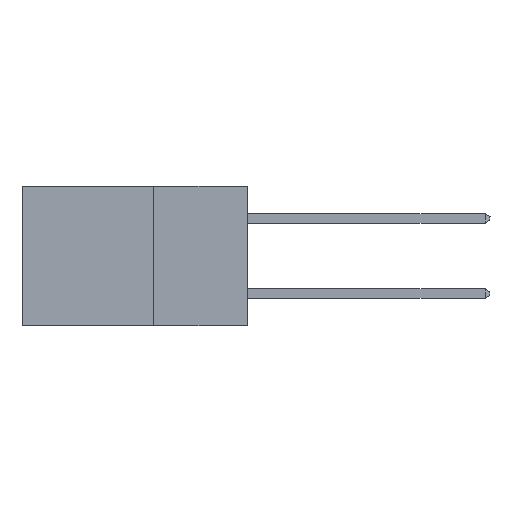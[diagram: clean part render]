
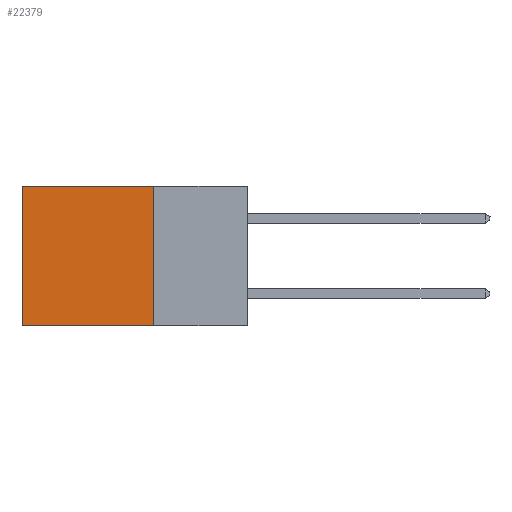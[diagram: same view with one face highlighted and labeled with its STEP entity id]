
A CAD part, left-side view. The second image highlights one B-rep face of the part: STEP entity #22379.
In plain terms, the highlighted planar face has unit normal (-1, 0, 0).
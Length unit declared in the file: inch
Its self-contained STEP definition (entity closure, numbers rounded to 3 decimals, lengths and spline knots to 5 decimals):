
#1244 = VERTEX_POINT ( 'NONE', #3478 ) ;
#1535 = DIRECTION ( 'NONE',  ( 0., 1., 0. ) ) ;
#2784 = AXIS2_PLACEMENT_3D ( 'NONE', #3380, #22066, #13731 ) ;
#3104 = EDGE_CURVE ( 'NONE', #1244, #11530, #9121, .T. ) ;
#3380 = CARTESIAN_POINT ( 'NONE',  ( 0.2615, 0.25, -0.37 ) ) ;
#3478 = CARTESIAN_POINT ( 'NONE',  ( 0.2615, 0.25, 0. ) ) ;
#4189 = DIRECTION ( 'NONE',  ( 0., 1., 0. ) ) ;
#4987 = LINE ( 'NONE', #11821, #6689 ) ;
#5303 = EDGE_LOOP ( 'NONE', ( #19051, #20896, #7259, #17029 ) ) ;
#5463 = DIRECTION ( 'NONE',  ( 0., 0., -1. ) ) ;
#6643 = LINE ( 'NONE', #10264, #13486 ) ;
#6689 = VECTOR ( 'NONE', #22068, 39.37008 ) ;
#7259 = ORIENTED_EDGE ( 'NONE', *, *, #3104, .F. ) ;
#7707 = LINE ( 'NONE', #18281, #16753 ) ;
#8409 = PLANE ( 'NONE',  #2784 ) ;
#8454 = CARTESIAN_POINT ( 'NONE',  ( 0.2615, 0.25, -0.37 ) ) ;
#8784 = CARTESIAN_POINT ( 'NONE',  ( 0.2615, 0.6, -0.37 ) ) ;
#8899 = EDGE_CURVE ( 'NONE', #11530, #14816, #6643, .T. ) ;
#9121 = LINE ( 'NONE', #12408, #9487 ) ;
#9487 = VECTOR ( 'NONE', #5463, 39.37008 ) ;
#10177 = EDGE_CURVE ( 'NONE', #1244, #15066, #7707, .T. ) ;
#10264 = CARTESIAN_POINT ( 'NONE',  ( 0.2615, 0.25, -0.37 ) ) ;
#11530 = VERTEX_POINT ( 'NONE', #8454 ) ;
#11821 = CARTESIAN_POINT ( 'NONE',  ( 0.2615, 0.6, -0.37 ) ) ;
#12408 = CARTESIAN_POINT ( 'NONE',  ( 0.2615, 0.25, -0.37 ) ) ;
#13486 = VECTOR ( 'NONE', #1535, 39.37008 ) ;
#13731 = DIRECTION ( 'NONE',  ( 0., 0., -1. ) ) ;
#13841 = FACE_OUTER_BOUND ( 'NONE', #5303, .T. ) ;
#14816 = VERTEX_POINT ( 'NONE', #8784 ) ;
#15066 = VERTEX_POINT ( 'NONE', #16134 ) ;
#16134 = CARTESIAN_POINT ( 'NONE',  ( 0.2615, 0.6, 0. ) ) ;
#16753 = VECTOR ( 'NONE', #4189, 39.37008 ) ;
#17029 = ORIENTED_EDGE ( 'NONE', *, *, #10177, .T. ) ;
#18094 = EDGE_CURVE ( 'NONE', #15066, #14816, #4987, .T. ) ;
#18281 = CARTESIAN_POINT ( 'NONE',  ( 0.2615, 0.25, 0. ) ) ;
#19051 = ORIENTED_EDGE ( 'NONE', *, *, #18094, .T. ) ;
#20896 = ORIENTED_EDGE ( 'NONE', *, *, #8899, .F. ) ;
#22066 = DIRECTION ( 'NONE',  ( 1., 0., 0. ) ) ;
#22068 = DIRECTION ( 'NONE',  ( 0., 0., -1. ) ) ;
#22379 = ADVANCED_FACE ( 'NONE', ( #13841 ), #8409, .F. ) ;
